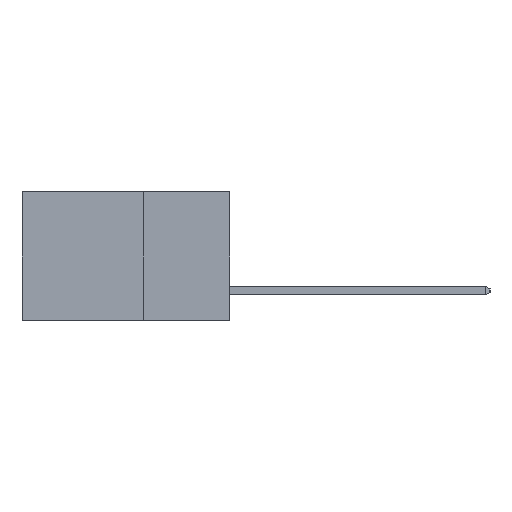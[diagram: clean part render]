
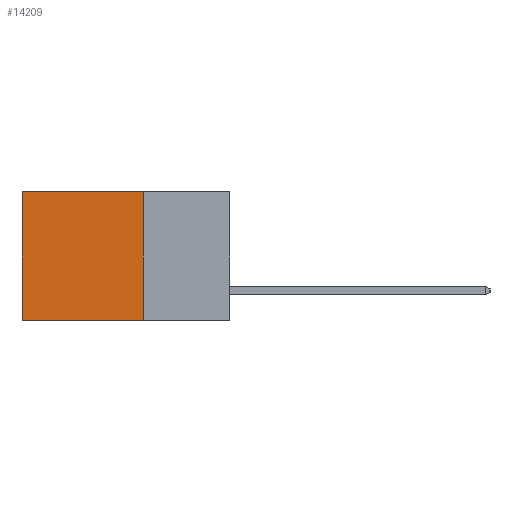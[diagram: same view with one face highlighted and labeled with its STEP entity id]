
A CAD part, left-side view. The second image highlights one B-rep face of the part: STEP entity #14209.
In plain terms, the highlighted planar face has unit normal (-1, 0, 0).
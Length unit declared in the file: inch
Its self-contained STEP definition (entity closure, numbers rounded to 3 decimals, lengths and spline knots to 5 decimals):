
#59 = CARTESIAN_POINT ( 'NONE',  ( 0.2615, 0.25, -0.37 ) ) ;
#616 = LINE ( 'NONE', #6272, #10151 ) ;
#1186 = EDGE_CURVE ( 'NONE', #7224, #3007, #8746, .T. ) ;
#1200 = ORIENTED_EDGE ( 'NONE', *, *, #7025, .F. ) ;
#2216 = CARTESIAN_POINT ( 'NONE',  ( 0.2615, 0.25, -0.37 ) ) ;
#3007 = VERTEX_POINT ( 'NONE', #13897 ) ;
#3280 = DIRECTION ( 'NONE',  ( 0., 0., -1. ) ) ;
#3565 = DIRECTION ( 'NONE',  ( 0., 1., 0. ) ) ;
#3925 = EDGE_LOOP ( 'NONE', ( #7075, #1200, #12958, #6767 ) ) ;
#4170 = CARTESIAN_POINT ( 'NONE',  ( 0.2615, 0.6, -0.37 ) ) ;
#4389 = CARTESIAN_POINT ( 'NONE',  ( 0.2615, 0.25, 0. ) ) ;
#4442 = PLANE ( 'NONE',  #14126 ) ;
#4459 = FACE_OUTER_BOUND ( 'NONE', #3925, .T. ) ;
#5346 = CARTESIAN_POINT ( 'NONE',  ( 0.2615, 0.25, -0.37 ) ) ;
#5375 = VERTEX_POINT ( 'NONE', #4170 ) ;
#5993 = EDGE_CURVE ( 'NONE', #7224, #8390, #10846, .T. ) ;
#6272 = CARTESIAN_POINT ( 'NONE',  ( 0.2615, 0.6, -0.37 ) ) ;
#6767 = ORIENTED_EDGE ( 'NONE', *, *, #1186, .T. ) ;
#7025 = EDGE_CURVE ( 'NONE', #8390, #5375, #15048, .T. ) ;
#7075 = ORIENTED_EDGE ( 'NONE', *, *, #11476, .T. ) ;
#7199 = DIRECTION ( 'NONE',  ( 0., 1., 0. ) ) ;
#7224 = VERTEX_POINT ( 'NONE', #4389 ) ;
#8062 = VECTOR ( 'NONE', #8927, 39.37008 ) ;
#8390 = VERTEX_POINT ( 'NONE', #59 ) ;
#8746 = LINE ( 'NONE', #15457, #9114 ) ;
#8927 = DIRECTION ( 'NONE',  ( 0., 0., -1. ) ) ;
#9114 = VECTOR ( 'NONE', #7199, 39.37008 ) ;
#10151 = VECTOR ( 'NONE', #13413, 39.37008 ) ;
#10519 = DIRECTION ( 'NONE',  ( 1., 0., 0. ) ) ;
#10846 = LINE ( 'NONE', #5346, #8062 ) ;
#11476 = EDGE_CURVE ( 'NONE', #3007, #5375, #616, .T. ) ;
#11909 = VECTOR ( 'NONE', #3565, 39.37008 ) ;
#12833 = CARTESIAN_POINT ( 'NONE',  ( 0.2615, 0.25, -0.37 ) ) ;
#12958 = ORIENTED_EDGE ( 'NONE', *, *, #5993, .F. ) ;
#13413 = DIRECTION ( 'NONE',  ( 0., 0., -1. ) ) ;
#13897 = CARTESIAN_POINT ( 'NONE',  ( 0.2615, 0.6, 0. ) ) ;
#14126 = AXIS2_PLACEMENT_3D ( 'NONE', #12833, #10519, #3280 ) ;
#14209 = ADVANCED_FACE ( 'NONE', ( #4459 ), #4442, .F. ) ;
#15048 = LINE ( 'NONE', #2216, #11909 ) ;
#15457 = CARTESIAN_POINT ( 'NONE',  ( 0.2615, 0.25, 0. ) ) ;
